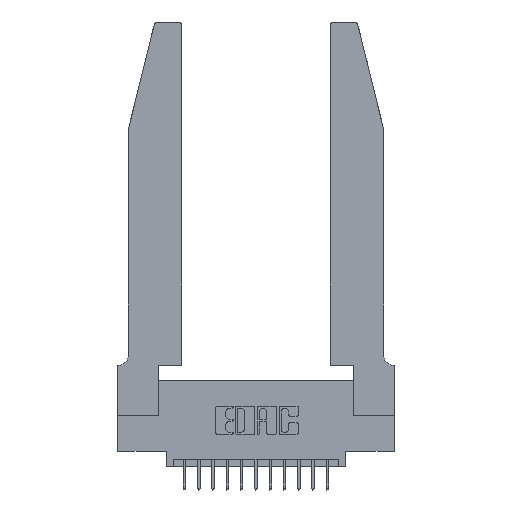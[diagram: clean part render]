
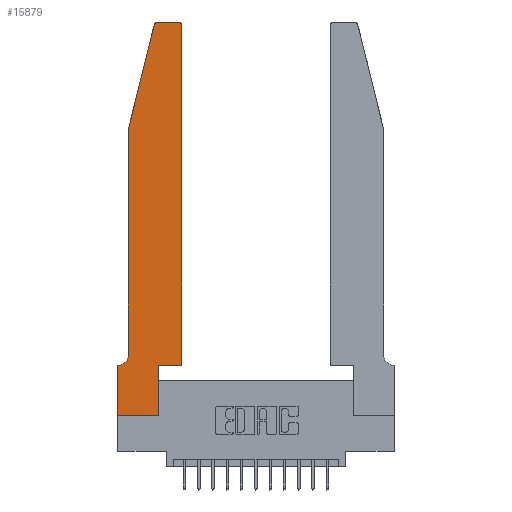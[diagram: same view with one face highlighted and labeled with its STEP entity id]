
A CAD part, top view. The second image highlights one B-rep face of the part: STEP entity #15879.
In plain terms, the highlighted planar face has unit normal (0, 0, 1).
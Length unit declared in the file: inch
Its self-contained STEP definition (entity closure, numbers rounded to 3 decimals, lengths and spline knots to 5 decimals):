
#210 = EDGE_CURVE ( 'NONE', #3461, #7142, #5548, .T. ) ;
#229 = EDGE_CURVE ( 'NONE', #5433, #6878, #12423, .T. ) ;
#552 = EDGE_CURVE ( 'NONE', #17567, #14846, #8768, .T. ) ;
#735 = VERTEX_POINT ( 'NONE', #11688 ) ;
#1005 = CARTESIAN_POINT ( 'NONE',  ( 0.0755, 0.42, 0.37 ) ) ;
#1661 = EDGE_CURVE ( 'NONE', #6878, #4642, #3962, .T. ) ;
#1735 = DIRECTION ( 'NONE',  ( -1., 0., 0. ) ) ;
#1931 = DIRECTION ( 'NONE',  ( 1., 0., 0. ) ) ;
#1947 = ORIENTED_EDGE ( 'NONE', *, *, #16009, .T. ) ;
#2109 = CARTESIAN_POINT ( 'NONE',  ( 0.284, 2.72, 0.37 ) ) ;
#2220 = DIRECTION ( 'NONE',  ( 0., 0., 1. ) ) ;
#2437 = EDGE_CURVE ( 'NONE', #2526, #9601, #13866, .T. ) ;
#2526 = VERTEX_POINT ( 'NONE', #9046 ) ;
#2656 = VECTOR ( 'NONE', #12868, 39.37008 ) ;
#2722 = ORIENTED_EDGE ( 'NONE', *, *, #229, .T. ) ;
#2970 = CARTESIAN_POINT ( 'NONE',  ( 0.2865, 0.35, 0.37 ) ) ;
#3153 = VECTOR ( 'NONE', #8432, 39.37008 ) ;
#3285 = LINE ( 'NONE', #2970, #2656 ) ;
#3326 = ORIENTED_EDGE ( 'NONE', *, *, #15435, .T. ) ;
#3461 = VERTEX_POINT ( 'NONE', #11256 ) ;
#3832 = CARTESIAN_POINT ( 'NONE',  ( 0.4505, 0.35, 0.37 ) ) ;
#3962 = CIRCLE ( 'NONE', #7085, 0.03 ) ;
#4315 = EDGE_CURVE ( 'NONE', #4780, #2526, #9808, .T. ) ;
#4495 = VERTEX_POINT ( 'NONE', #13969 ) ;
#4642 = VERTEX_POINT ( 'NONE', #8950 ) ;
#4706 = EDGE_CURVE ( 'NONE', #735, #4780, #3285, .T. ) ;
#4780 = VERTEX_POINT ( 'NONE', #14408 ) ;
#5433 = VERTEX_POINT ( 'NONE', #9252 ) ;
#5548 = LINE ( 'NONE', #16777, #7928 ) ;
#5606 = ORIENTED_EDGE ( 'NONE', *, *, #210, .T. ) ;
#5682 = DIRECTION ( 'NONE',  ( 0., 0., 1. ) ) ;
#5730 = AXIS2_PLACEMENT_3D ( 'NONE', #7262, #5682, #11148 ) ;
#5757 = CARTESIAN_POINT ( 'NONE',  ( 0.4505, 0.35, 0.37 ) ) ;
#5771 = ORIENTED_EDGE ( 'NONE', *, *, #10590, .T. ) ;
#5941 = PLANE ( 'NONE',  #5730 ) ;
#6022 = DIRECTION ( 'NONE',  ( -0.239, -0.971, 0. ) ) ;
#6365 = ORIENTED_EDGE ( 'NONE', *, *, #2437, .T. ) ;
#6510 = CARTESIAN_POINT ( 'NONE',  ( 0.0755, 2., 0.37 ) ) ;
#6583 = EDGE_CURVE ( 'NONE', #4495, #735, #10189, .T. ) ;
#6655 = DIRECTION ( 'NONE',  ( 1., 0., 0. ) ) ;
#6878 = VERTEX_POINT ( 'NONE', #12040 ) ;
#7085 = AXIS2_PLACEMENT_3D ( 'NONE', #2109, #2220, #10315 ) ;
#7142 = VERTEX_POINT ( 'NONE', #12328 ) ;
#7262 = CARTESIAN_POINT ( 'NONE',  ( 0., 0.35, 0.37 ) ) ;
#7917 = AXIS2_PLACEMENT_3D ( 'NONE', #12422, #8227, #16276 ) ;
#7925 = CARTESIAN_POINT ( 'NONE',  ( 0.0755, 2., 0.37 ) ) ;
#7928 = VECTOR ( 'NONE', #1735, 39.37008 ) ;
#8114 = LINE ( 'NONE', #11467, #12376 ) ;
#8227 = DIRECTION ( 'NONE',  ( 0., 0., -1. ) ) ;
#8432 = DIRECTION ( 'NONE',  ( -1., 0., 0. ) ) ;
#8768 = LINE ( 'NONE', #6510, #15644 ) ;
#8817 = ORIENTED_EDGE ( 'NONE', *, *, #6583, .T. ) ;
#8950 = CARTESIAN_POINT ( 'NONE',  ( 0.25487, 2.72718, 0.37 ) ) ;
#9046 = CARTESIAN_POINT ( 'NONE',  ( 0.4505, 0.35, 0.37 ) ) ;
#9176 = EDGE_LOOP ( 'NONE', ( #2722, #17150, #3326, #16425, #14594, #5606, #5771, #8817, #11782, #11537, #6365, #1947 ) ) ;
#9252 = CARTESIAN_POINT ( 'NONE',  ( 0.4205, 2.75, 0.37 ) ) ;
#9289 = CARTESIAN_POINT ( 'NONE',  ( 0., 0., 0.37 ) ) ;
#9601 = VERTEX_POINT ( 'NONE', #14853 ) ;
#9789 = DIRECTION ( 'NONE',  ( 0., 1., 0. ) ) ;
#9808 = LINE ( 'NONE', #3832, #14313 ) ;
#9823 = CIRCLE ( 'NONE', #10912, 0.03 ) ;
#9827 = DIRECTION ( 'NONE',  ( 0., -1., 0. ) ) ;
#10189 = LINE ( 'NONE', #9289, #15336 ) ;
#10198 = DIRECTION ( 'NONE',  ( 0., 0., 1. ) ) ;
#10315 = DIRECTION ( 'NONE',  ( 1., 0., 0. ) ) ;
#10590 = EDGE_CURVE ( 'NONE', #7142, #4495, #16412, .T. ) ;
#10845 = VECTOR ( 'NONE', #9827, 39.37008 ) ;
#10912 = AXIS2_PLACEMENT_3D ( 'NONE', #14444, #10198, #1931 ) ;
#11148 = DIRECTION ( 'NONE',  ( 1., 0., 0. ) ) ;
#11256 = CARTESIAN_POINT ( 'NONE',  ( 0.0055, 0.35, 0.37 ) ) ;
#11467 = CARTESIAN_POINT ( 'NONE',  ( 0.0755, 2., 0.37 ) ) ;
#11537 = ORIENTED_EDGE ( 'NONE', *, *, #4315, .T. ) ;
#11688 = CARTESIAN_POINT ( 'NONE',  ( 0.2865, 0., 0.37 ) ) ;
#11782 = ORIENTED_EDGE ( 'NONE', *, *, #4706, .T. ) ;
#12040 = CARTESIAN_POINT ( 'NONE',  ( 0.284, 2.75, 0.37 ) ) ;
#12328 = CARTESIAN_POINT ( 'NONE',  ( 0., 0.35, 0.37 ) ) ;
#12376 = VECTOR ( 'NONE', #6022, 39.37008 ) ;
#12422 = CARTESIAN_POINT ( 'NONE',  ( 0.0055, 0.42, 0.37 ) ) ;
#12423 = LINE ( 'NONE', #16650, #3153 ) ;
#12773 = EDGE_CURVE ( 'NONE', #14846, #3461, #14438, .T. ) ;
#12868 = DIRECTION ( 'NONE',  ( 0., 1., 0. ) ) ;
#13866 = LINE ( 'NONE', #5757, #16648 ) ;
#13969 = CARTESIAN_POINT ( 'NONE',  ( 0., 0., 0.37 ) ) ;
#14068 = CARTESIAN_POINT ( 'NONE',  ( 0., 0., 0.37 ) ) ;
#14313 = VECTOR ( 'NONE', #15156, 39.37008 ) ;
#14408 = CARTESIAN_POINT ( 'NONE',  ( 0.2865, 0.35, 0.37 ) ) ;
#14438 = CIRCLE ( 'NONE', #7917, 0.07 ) ;
#14444 = CARTESIAN_POINT ( 'NONE',  ( 0.4205, 2.72, 0.37 ) ) ;
#14594 = ORIENTED_EDGE ( 'NONE', *, *, #12773, .T. ) ;
#14846 = VERTEX_POINT ( 'NONE', #1005 ) ;
#14853 = CARTESIAN_POINT ( 'NONE',  ( 0.4505, 2.72, 0.37 ) ) ;
#15156 = DIRECTION ( 'NONE',  ( 1., 0., 0. ) ) ;
#15336 = VECTOR ( 'NONE', #6655, 39.37008 ) ;
#15435 = EDGE_CURVE ( 'NONE', #4642, #17567, #8114, .T. ) ;
#15644 = VECTOR ( 'NONE', #17473, 39.37008 ) ;
#15879 = ADVANCED_FACE ( 'NONE', ( #17536 ), #5941, .T. ) ;
#16009 = EDGE_CURVE ( 'NONE', #9601, #5433, #9823, .T. ) ;
#16276 = DIRECTION ( 'NONE',  ( -1., 0., 0. ) ) ;
#16412 = LINE ( 'NONE', #14068, #10845 ) ;
#16425 = ORIENTED_EDGE ( 'NONE', *, *, #552, .T. ) ;
#16648 = VECTOR ( 'NONE', #9789, 39.37008 ) ;
#16650 = CARTESIAN_POINT ( 'NONE',  ( 0.2605, 2.75, 0.37 ) ) ;
#16777 = CARTESIAN_POINT ( 'NONE',  ( 0.0755, 0.35, 0.37 ) ) ;
#17150 = ORIENTED_EDGE ( 'NONE', *, *, #1661, .T. ) ;
#17473 = DIRECTION ( 'NONE',  ( 0., -1., 0. ) ) ;
#17536 = FACE_OUTER_BOUND ( 'NONE', #9176, .T. ) ;
#17567 = VERTEX_POINT ( 'NONE', #7925 ) ;
